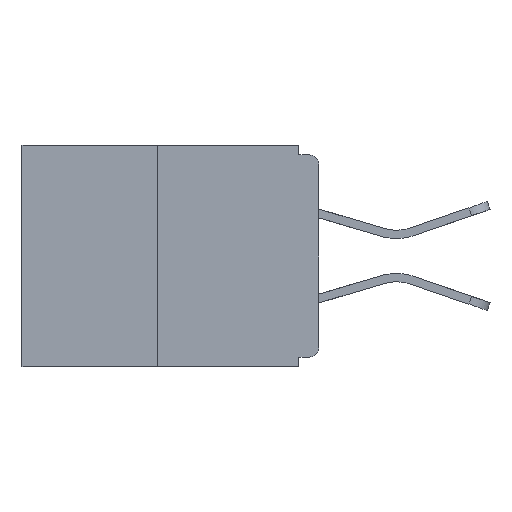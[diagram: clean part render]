
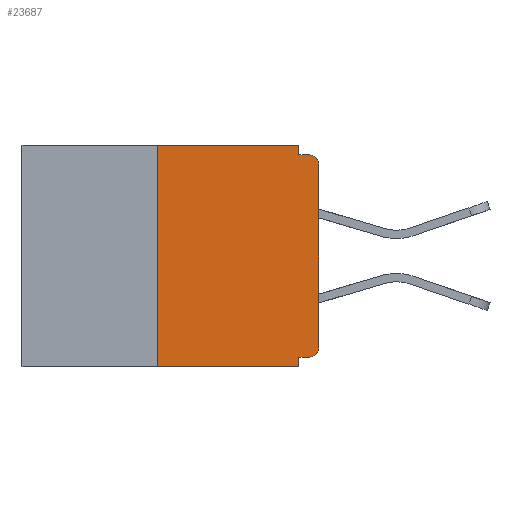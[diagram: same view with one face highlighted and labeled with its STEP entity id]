
A CAD part, left-side view. The second image highlights one B-rep face of the part: STEP entity #23687.
In plain terms, the highlighted planar face has unit normal (-1, 0, 0).
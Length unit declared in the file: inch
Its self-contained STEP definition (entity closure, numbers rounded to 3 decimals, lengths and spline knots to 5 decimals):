
#329 = FACE_OUTER_BOUND ( 'NONE', #22427, .T. ) ;
#415 = LINE ( 'NONE', #13769, #1331 ) ;
#1192 = EDGE_CURVE ( 'NONE', #13747, #11272, #17167, .T. ) ;
#1331 = VECTOR ( 'NONE', #4137, 39.37008 ) ;
#1346 = VECTOR ( 'NONE', #23461, 39.37008 ) ;
#1772 = VERTEX_POINT ( 'NONE', #13448 ) ;
#1951 = ORIENTED_EDGE ( 'NONE', *, *, #3154, .F. ) ;
#2160 = CARTESIAN_POINT ( 'NONE',  ( 0., 0., -0.328 ) ) ;
#2171 = EDGE_CURVE ( 'NONE', #15206, #1772, #24405, .T. ) ;
#2379 = PLANE ( 'NONE',  #10609 ) ;
#3129 = VERTEX_POINT ( 'NONE', #21267 ) ;
#3154 = EDGE_CURVE ( 'NONE', #19881, #13747, #16184, .T. ) ;
#3867 = VERTEX_POINT ( 'NONE', #11559 ) ;
#3891 = CARTESIAN_POINT ( 'NONE',  ( 0., 0.031, 0. ) ) ;
#4004 = CIRCLE ( 'NONE', #4345, 0.015 ) ;
#4047 = CARTESIAN_POINT ( 'NONE',  ( 0., 0.031, 0. ) ) ;
#4077 = DIRECTION ( 'NONE',  ( -1., 0., 0. ) ) ;
#4137 = DIRECTION ( 'NONE',  ( 0., 0., 1. ) ) ;
#4345 = AXIS2_PLACEMENT_3D ( 'NONE', #24821, #16986, #14964 ) ;
#4743 = ORIENTED_EDGE ( 'NONE', *, *, #16177, .F. ) ;
#5157 = LINE ( 'NONE', #19858, #9068 ) ;
#5666 = AXIS2_PLACEMENT_3D ( 'NONE', #25024, #4077, #5855 ) ;
#5855 = DIRECTION ( 'NONE',  ( 0., 0., -1. ) ) ;
#5865 = EDGE_CURVE ( 'NONE', #3867, #21333, #5157, .T. ) ;
#6150 = ORIENTED_EDGE ( 'NONE', *, *, #5865, .T. ) ;
#6280 = CARTESIAN_POINT ( 'NONE',  ( 0., 0.46, 0. ) ) ;
#6676 = CARTESIAN_POINT ( 'NONE',  ( 0., 0.46, -0.343 ) ) ;
#7022 = ORIENTED_EDGE ( 'NONE', *, *, #21923, .F. ) ;
#7282 = LINE ( 'NONE', #14532, #23961 ) ;
#8194 = ORIENTED_EDGE ( 'NONE', *, *, #2171, .F. ) ;
#8358 = ORIENTED_EDGE ( 'NONE', *, *, #1192, .F. ) ;
#9068 = VECTOR ( 'NONE', #10099, 39.37008 ) ;
#10099 = DIRECTION ( 'NONE',  ( 0., 0., 1. ) ) ;
#10238 = DIRECTION ( 'NONE',  ( 0., 0., -1. ) ) ;
#10609 = AXIS2_PLACEMENT_3D ( 'NONE', #6280, #15792, #17862 ) ;
#10713 = CARTESIAN_POINT ( 'NONE',  ( 0., 0.015, -0.015 ) ) ;
#10980 = EDGE_CURVE ( 'NONE', #19583, #1772, #19114, .T. ) ;
#11079 = CIRCLE ( 'NONE', #5666, 0.015 ) ;
#11272 = VERTEX_POINT ( 'NONE', #14283 ) ;
#11283 = EDGE_CURVE ( 'NONE', #11272, #22699, #7282, .T. ) ;
#11559 = CARTESIAN_POINT ( 'NONE',  ( 0., 0., -0.313 ) ) ;
#12837 = EDGE_CURVE ( 'NONE', #3129, #3867, #4004, .T. ) ;
#13448 = CARTESIAN_POINT ( 'NONE',  ( 0., 0.031, -0.343 ) ) ;
#13747 = VERTEX_POINT ( 'NONE', #3891 ) ;
#13769 = CARTESIAN_POINT ( 'NONE',  ( 0., 0.25, 0. ) ) ;
#13800 = ORIENTED_EDGE ( 'NONE', *, *, #11283, .F. ) ;
#14283 = CARTESIAN_POINT ( 'NONE',  ( 0., 0.031, -0.015 ) ) ;
#14532 = CARTESIAN_POINT ( 'NONE',  ( 0., 0., -0.015 ) ) ;
#14950 = VECTOR ( 'NONE', #15520, 39.37008 ) ;
#14964 = DIRECTION ( 'NONE',  ( 0., 0., -1. ) ) ;
#15206 = VERTEX_POINT ( 'NONE', #18425 ) ;
#15289 = EDGE_CURVE ( 'NONE', #21333, #22699, #11079, .T. ) ;
#15520 = DIRECTION ( 'NONE',  ( 0., -1., 0. ) ) ;
#15792 = DIRECTION ( 'NONE',  ( 1., 0., 0. ) ) ;
#16177 = EDGE_CURVE ( 'NONE', #3129, #15206, #18640, .T. ) ;
#16184 = LINE ( 'NONE', #23413, #14950 ) ;
#16593 = CARTESIAN_POINT ( 'NONE',  ( 0., 0.25, 0. ) ) ;
#16986 = DIRECTION ( 'NONE',  ( -1., 0., 0. ) ) ;
#17167 = LINE ( 'NONE', #4047, #20780 ) ;
#17288 = VECTOR ( 'NONE', #17939, 39.37008 ) ;
#17301 = DIRECTION ( 'NONE',  ( 0., 0., -1. ) ) ;
#17722 = CARTESIAN_POINT ( 'NONE',  ( 0., 0.031, -0.343 ) ) ;
#17862 = DIRECTION ( 'NONE',  ( 0., 0., -1. ) ) ;
#17939 = DIRECTION ( 'NONE',  ( 0., -1., 0. ) ) ;
#18138 = DIRECTION ( 'NONE',  ( 0., -1., 0. ) ) ;
#18425 = CARTESIAN_POINT ( 'NONE',  ( 0., 0.031, -0.328 ) ) ;
#18640 = LINE ( 'NONE', #2160, #1346 ) ;
#19114 = LINE ( 'NONE', #6676, #17288 ) ;
#19583 = VERTEX_POINT ( 'NONE', #21108 ) ;
#19858 = CARTESIAN_POINT ( 'NONE',  ( 0., 0., 0. ) ) ;
#19881 = VERTEX_POINT ( 'NONE', #16593 ) ;
#20780 = VECTOR ( 'NONE', #17301, 39.37008 ) ;
#21108 = CARTESIAN_POINT ( 'NONE',  ( 0., 0.25, -0.343 ) ) ;
#21267 = CARTESIAN_POINT ( 'NONE',  ( 0., 0.015, -0.328 ) ) ;
#21333 = VERTEX_POINT ( 'NONE', #22137 ) ;
#21825 = ORIENTED_EDGE ( 'NONE', *, *, #10980, .T. ) ;
#21923 = EDGE_CURVE ( 'NONE', #19583, #19881, #415, .T. ) ;
#21989 = VECTOR ( 'NONE', #10238, 39.37008 ) ;
#22137 = CARTESIAN_POINT ( 'NONE',  ( 0., 0., -0.03 ) ) ;
#22232 = ORIENTED_EDGE ( 'NONE', *, *, #15289, .T. ) ;
#22427 = EDGE_LOOP ( 'NONE', ( #1951, #7022, #21825, #8194, #4743, #24118, #6150, #22232, #13800, #8358 ) ) ;
#22699 = VERTEX_POINT ( 'NONE', #10713 ) ;
#23413 = CARTESIAN_POINT ( 'NONE',  ( 0., 0.46, 0. ) ) ;
#23461 = DIRECTION ( 'NONE',  ( 0., 1., 0. ) ) ;
#23687 = ADVANCED_FACE ( 'NONE', ( #329 ), #2379, .F. ) ;
#23961 = VECTOR ( 'NONE', #18138, 39.37008 ) ;
#24118 = ORIENTED_EDGE ( 'NONE', *, *, #12837, .T. ) ;
#24405 = LINE ( 'NONE', #17722, #21989 ) ;
#24821 = CARTESIAN_POINT ( 'NONE',  ( 0., 0.015, -0.313 ) ) ;
#25024 = CARTESIAN_POINT ( 'NONE',  ( 0., 0.015, -0.03 ) ) ;
